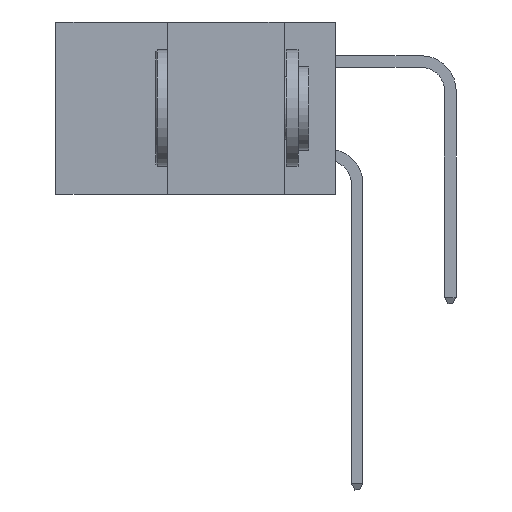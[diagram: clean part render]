
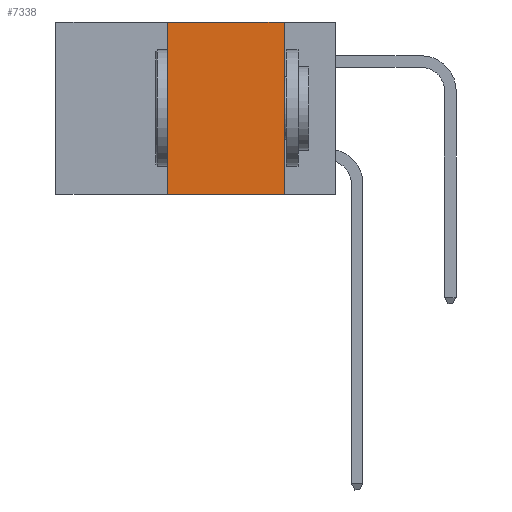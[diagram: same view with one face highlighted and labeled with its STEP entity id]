
A CAD part, left-side view. The second image highlights one B-rep face of the part: STEP entity #7338.
In plain terms, the highlighted planar face has unit normal (-1, 0, 0).
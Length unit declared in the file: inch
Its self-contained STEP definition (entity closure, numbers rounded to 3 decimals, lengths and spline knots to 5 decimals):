
#941 = VERTEX_POINT ( 'NONE', #28396 ) ;
#4313 = CARTESIAN_POINT ( 'NONE',  ( 0., 0.6, -0.37 ) ) ;
#4645 = VERTEX_POINT ( 'NONE', #16477 ) ;
#5176 = LINE ( 'NONE', #13653, #14480 ) ;
#5623 = CARTESIAN_POINT ( 'NONE',  ( 0., 0.11, 0. ) ) ;
#7338 = ADVANCED_FACE ( 'NONE', ( #24799 ), #14180, .F. ) ;
#7549 = EDGE_LOOP ( 'NONE', ( #39474, #24935, #9889, #37092 ) ) ;
#8788 = EDGE_CURVE ( 'NONE', #941, #40501, #14598, .T. ) ;
#8821 = CARTESIAN_POINT ( 'NONE',  ( 0., 0.11, 0. ) ) ;
#9547 = EDGE_CURVE ( 'NONE', #30968, #40501, #20941, .T. ) ;
#9889 = ORIENTED_EDGE ( 'NONE', *, *, #29167, .F. ) ;
#10091 = EDGE_CURVE ( 'NONE', #4645, #30968, #5176, .T. ) ;
#10231 = AXIS2_PLACEMENT_3D ( 'NONE', #30583, #26111, #11285 ) ;
#11285 = DIRECTION ( 'NONE',  ( 0., 0., -1. ) ) ;
#13653 = CARTESIAN_POINT ( 'NONE',  ( 0., 0.6, 0. ) ) ;
#14180 = PLANE ( 'NONE',  #10231 ) ;
#14480 = VECTOR ( 'NONE', #20120, 39.37008 ) ;
#14598 = LINE ( 'NONE', #4313, #21984 ) ;
#16477 = CARTESIAN_POINT ( 'NONE',  ( 0., 0.36, 0. ) ) ;
#19921 = VECTOR ( 'NONE', #31615, 39.37008 ) ;
#20120 = DIRECTION ( 'NONE',  ( 0., -1., 0. ) ) ;
#20415 = CARTESIAN_POINT ( 'NONE',  ( 0., 0.36, 0. ) ) ;
#20941 = LINE ( 'NONE', #5623, #19921 ) ;
#21984 = VECTOR ( 'NONE', #25790, 39.37008 ) ;
#24657 = CARTESIAN_POINT ( 'NONE',  ( 0., 0.11, -0.37 ) ) ;
#24799 = FACE_OUTER_BOUND ( 'NONE', #7549, .T. ) ;
#24935 = ORIENTED_EDGE ( 'NONE', *, *, #10091, .F. ) ;
#25790 = DIRECTION ( 'NONE',  ( 0., -1., 0. ) ) ;
#26001 = LINE ( 'NONE', #20415, #39777 ) ;
#26111 = DIRECTION ( 'NONE',  ( 1., 0., 0. ) ) ;
#28396 = CARTESIAN_POINT ( 'NONE',  ( 0., 0.36, -0.37 ) ) ;
#29167 = EDGE_CURVE ( 'NONE', #941, #4645, #26001, .T. ) ;
#30583 = CARTESIAN_POINT ( 'NONE',  ( 0., 0.6, 0. ) ) ;
#30968 = VERTEX_POINT ( 'NONE', #8821 ) ;
#31615 = DIRECTION ( 'NONE',  ( 0., 0., -1. ) ) ;
#35611 = DIRECTION ( 'NONE',  ( 0., 0., 1. ) ) ;
#37092 = ORIENTED_EDGE ( 'NONE', *, *, #8788, .T. ) ;
#39474 = ORIENTED_EDGE ( 'NONE', *, *, #9547, .F. ) ;
#39777 = VECTOR ( 'NONE', #35611, 39.37008 ) ;
#40501 = VERTEX_POINT ( 'NONE', #24657 ) ;
